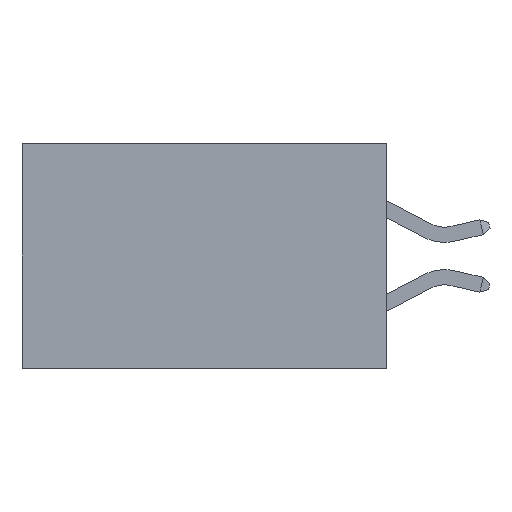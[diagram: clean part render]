
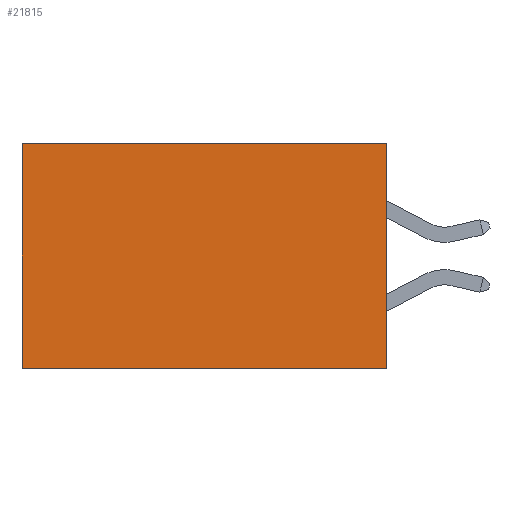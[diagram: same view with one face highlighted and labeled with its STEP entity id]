
A CAD part, left-side view. The second image highlights one B-rep face of the part: STEP entity #21815.
In plain terms, the highlighted planar face has unit normal (-1, 0, 0).
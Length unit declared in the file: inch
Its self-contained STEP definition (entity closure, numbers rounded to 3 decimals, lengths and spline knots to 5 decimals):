
#114 = ORIENTED_EDGE ( 'NONE', *, *, #2917, .F. ) ;
#122 = VERTEX_POINT ( 'NONE', #5092 ) ;
#358 = ORIENTED_EDGE ( 'NONE', *, *, #22146, .F. ) ;
#821 = ORIENTED_EDGE ( 'NONE', *, *, #24889, .T. ) ;
#1199 = AXIS2_PLACEMENT_3D ( 'NONE', #7963, #16332, #3797 ) ;
#1253 = CARTESIAN_POINT ( 'NONE',  ( 0.298, 0.6, 0. ) ) ;
#1376 = VERTEX_POINT ( 'NONE', #2646 ) ;
#1815 = EDGE_CURVE ( 'NONE', #122, #1376, #6062, .T. ) ;
#2359 = CARTESIAN_POINT ( 'NONE',  ( 0.298, 0.6, -0.37 ) ) ;
#2646 = CARTESIAN_POINT ( 'NONE',  ( 0.298, 0.6, 0. ) ) ;
#2917 = EDGE_CURVE ( 'NONE', #15920, #12439, #22732, .T. ) ;
#3797 = DIRECTION ( 'NONE',  ( 0., 0., -1. ) ) ;
#3915 = VECTOR ( 'NONE', #15247, 39.37008 ) ;
#4576 = LINE ( 'NONE', #21311, #3915 ) ;
#5092 = CARTESIAN_POINT ( 'NONE',  ( 0.298, 0., 0. ) ) ;
#6062 = LINE ( 'NONE', #9618, #16500 ) ;
#7616 = DIRECTION ( 'NONE',  ( 0., 0., -1. ) ) ;
#7963 = CARTESIAN_POINT ( 'NONE',  ( 0.298, 0., 0. ) ) ;
#8306 = VECTOR ( 'NONE', #13533, 39.37008 ) ;
#9618 = CARTESIAN_POINT ( 'NONE',  ( 0.298, 0., 0. ) ) ;
#12439 = VERTEX_POINT ( 'NONE', #2359 ) ;
#13337 = DIRECTION ( 'NONE',  ( 0., 1., 0. ) ) ;
#13533 = DIRECTION ( 'NONE',  ( 0., 1., 0. ) ) ;
#14295 = PLANE ( 'NONE',  #1199 ) ;
#15247 = DIRECTION ( 'NONE',  ( 0., 0., -1. ) ) ;
#15327 = CARTESIAN_POINT ( 'NONE',  ( 0.298, 0., -0.37 ) ) ;
#15920 = VERTEX_POINT ( 'NONE', #16379 ) ;
#16332 = DIRECTION ( 'NONE',  ( 1., 0., 0. ) ) ;
#16379 = CARTESIAN_POINT ( 'NONE',  ( 0.298, 0., -0.37 ) ) ;
#16500 = VECTOR ( 'NONE', #13337, 39.37008 ) ;
#16685 = FACE_OUTER_BOUND ( 'NONE', #25603, .T. ) ;
#19962 = VECTOR ( 'NONE', #7616, 39.37008 ) ;
#21311 = CARTESIAN_POINT ( 'NONE',  ( 0.298, 0., 0. ) ) ;
#21815 = ADVANCED_FACE ( 'NONE', ( #16685 ), #14295, .F. ) ;
#22146 = EDGE_CURVE ( 'NONE', #122, #15920, #4576, .T. ) ;
#22732 = LINE ( 'NONE', #15327, #8306 ) ;
#24236 = ORIENTED_EDGE ( 'NONE', *, *, #1815, .T. ) ;
#24889 = EDGE_CURVE ( 'NONE', #1376, #12439, #25354, .T. ) ;
#25354 = LINE ( 'NONE', #1253, #19962 ) ;
#25603 = EDGE_LOOP ( 'NONE', ( #821, #114, #358, #24236 ) ) ;
